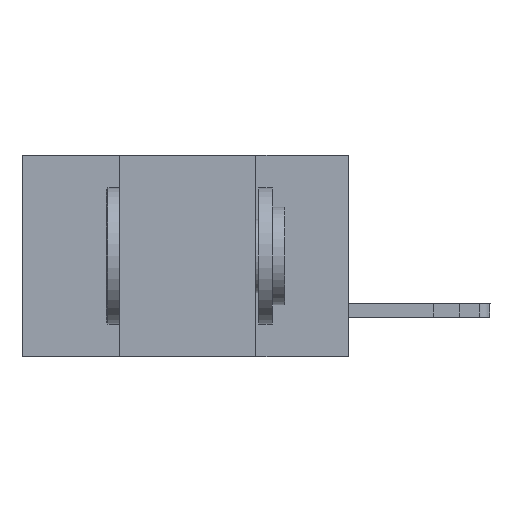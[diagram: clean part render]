
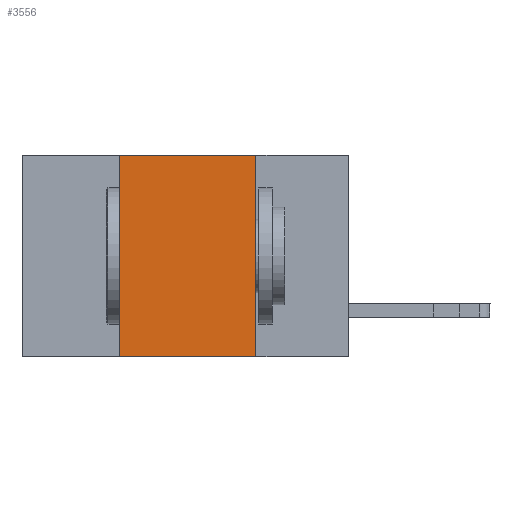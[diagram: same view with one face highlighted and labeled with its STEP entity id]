
A CAD part, left-side view. The second image highlights one B-rep face of the part: STEP entity #3556.
In plain terms, the highlighted planar face has unit normal (-1, 0, 0).
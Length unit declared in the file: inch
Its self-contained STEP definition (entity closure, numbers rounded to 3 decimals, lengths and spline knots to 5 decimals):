
#545 = DIRECTION ( 'NONE',  ( 0., 0., 1. ) ) ;
#601 = EDGE_CURVE ( 'NONE', #1891, #746, #945, .T. ) ;
#746 = VERTEX_POINT ( 'NONE', #3652 ) ;
#796 = CARTESIAN_POINT ( 'NONE',  ( 0., 0.6, -0.37 ) ) ;
#897 = FACE_OUTER_BOUND ( 'NONE', #1163, .T. ) ;
#945 = LINE ( 'NONE', #5034, #2308 ) ;
#966 = DIRECTION ( 'NONE',  ( 0., -1., 0. ) ) ;
#1163 = EDGE_LOOP ( 'NONE', ( #3592, #6142, #10048, #4605 ) ) ;
#1700 = LINE ( 'NONE', #796, #2388 ) ;
#1799 = EDGE_CURVE ( 'NONE', #8506, #2258, #1700, .T. ) ;
#1891 = VERTEX_POINT ( 'NONE', #7053 ) ;
#1985 = CARTESIAN_POINT ( 'NONE',  ( 0., 0.6, 0. ) ) ;
#2034 = CARTESIAN_POINT ( 'NONE',  ( 0., 0.17, -0.37 ) ) ;
#2258 = VERTEX_POINT ( 'NONE', #4532 ) ;
#2308 = VECTOR ( 'NONE', #3345, 39.37008 ) ;
#2388 = VECTOR ( 'NONE', #966, 39.37008 ) ;
#2909 = VECTOR ( 'NONE', #545, 39.37008 ) ;
#3293 = DIRECTION ( 'NONE',  ( 1., 0., 0. ) ) ;
#3345 = DIRECTION ( 'NONE',  ( 0., -1., 0. ) ) ;
#3556 = ADVANCED_FACE ( 'NONE', ( #897 ), #5727, .F. ) ;
#3592 = ORIENTED_EDGE ( 'NONE', *, *, #8143, .F. ) ;
#3652 = CARTESIAN_POINT ( 'NONE',  ( 0., 0.17, 0. ) ) ;
#3808 = LINE ( 'NONE', #2034, #4123 ) ;
#4123 = VECTOR ( 'NONE', #10333, 39.37008 ) ;
#4375 = DIRECTION ( 'NONE',  ( 0., 0., -1. ) ) ;
#4532 = CARTESIAN_POINT ( 'NONE',  ( 0., 0.17, -0.37 ) ) ;
#4605 = ORIENTED_EDGE ( 'NONE', *, *, #1799, .T. ) ;
#5034 = CARTESIAN_POINT ( 'NONE',  ( 0., 0.6, 0. ) ) ;
#5641 = CARTESIAN_POINT ( 'NONE',  ( 0., 0.42, -0.37 ) ) ;
#5727 = PLANE ( 'NONE',  #6839 ) ;
#6142 = ORIENTED_EDGE ( 'NONE', *, *, #601, .F. ) ;
#6839 = AXIS2_PLACEMENT_3D ( 'NONE', #1985, #3293, #4375 ) ;
#7053 = CARTESIAN_POINT ( 'NONE',  ( 0., 0.42, 0. ) ) ;
#7551 = EDGE_CURVE ( 'NONE', #8506, #1891, #8723, .T. ) ;
#8143 = EDGE_CURVE ( 'NONE', #746, #2258, #3808, .T. ) ;
#8506 = VERTEX_POINT ( 'NONE', #9962 ) ;
#8723 = LINE ( 'NONE', #5641, #2909 ) ;
#9962 = CARTESIAN_POINT ( 'NONE',  ( 0., 0.42, -0.37 ) ) ;
#10048 = ORIENTED_EDGE ( 'NONE', *, *, #7551, .F. ) ;
#10333 = DIRECTION ( 'NONE',  ( 0., 0., -1. ) ) ;
